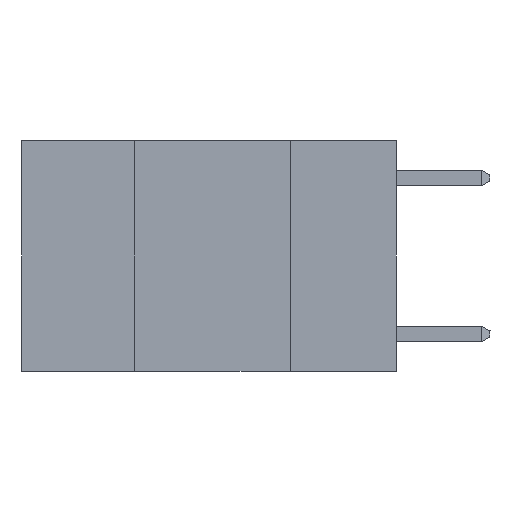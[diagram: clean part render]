
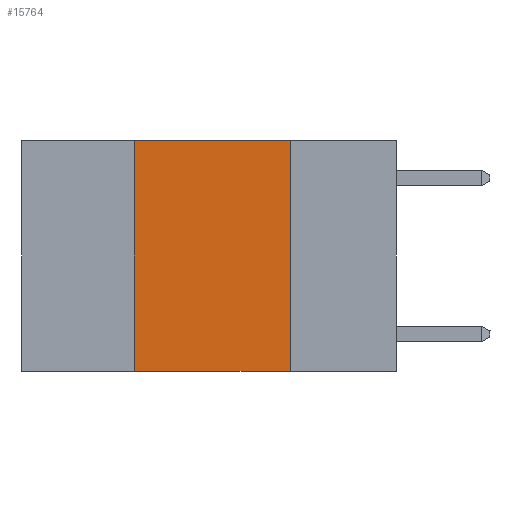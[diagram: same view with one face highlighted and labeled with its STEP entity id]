
A CAD part, left-side view. The second image highlights one B-rep face of the part: STEP entity #15764.
In plain terms, the highlighted planar face has unit normal (-1, 0, 0).
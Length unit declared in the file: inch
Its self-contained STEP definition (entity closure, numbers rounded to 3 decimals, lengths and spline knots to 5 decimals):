
#471 = CARTESIAN_POINT ( 'NONE',  ( 0., 0.6, 0. ) ) ;
#725 = VECTOR ( 'NONE', #10613, 39.37008 ) ;
#730 = VERTEX_POINT ( 'NONE', #13146 ) ;
#886 = CARTESIAN_POINT ( 'NONE',  ( 0., 0.6, -0.37 ) ) ;
#1570 = CARTESIAN_POINT ( 'NONE',  ( 0., 0.17, -0.37 ) ) ;
#1637 = ORIENTED_EDGE ( 'NONE', *, *, #3206, .T. ) ;
#1880 = CARTESIAN_POINT ( 'NONE',  ( 0., 0.17, 0. ) ) ;
#2827 = VERTEX_POINT ( 'NONE', #10248 ) ;
#3206 = EDGE_CURVE ( 'NONE', #8935, #9605, #15779, .T. ) ;
#3529 = DIRECTION ( 'NONE',  ( 0., 0., -1. ) ) ;
#4680 = FACE_OUTER_BOUND ( 'NONE', #5407, .T. ) ;
#5188 = CARTESIAN_POINT ( 'NONE',  ( 0., 0.42, 0. ) ) ;
#5199 = ORIENTED_EDGE ( 'NONE', *, *, #7371, .F. ) ;
#5407 = EDGE_LOOP ( 'NONE', ( #5199, #9253, #9108, #1637 ) ) ;
#5708 = DIRECTION ( 'NONE',  ( 0., 0., -1. ) ) ;
#6234 = DIRECTION ( 'NONE',  ( 0., -1., 0. ) ) ;
#6516 = LINE ( 'NONE', #5188, #725 ) ;
#7340 = DIRECTION ( 'NONE',  ( 1., 0., 0. ) ) ;
#7371 = EDGE_CURVE ( 'NONE', #730, #9605, #13830, .T. ) ;
#7540 = DIRECTION ( 'NONE',  ( 0., -1., 0. ) ) ;
#7768 = CARTESIAN_POINT ( 'NONE',  ( 0., 0.42, -0.37 ) ) ;
#8935 = VERTEX_POINT ( 'NONE', #7768 ) ;
#9108 = ORIENTED_EDGE ( 'NONE', *, *, #10853, .F. ) ;
#9253 = ORIENTED_EDGE ( 'NONE', *, *, #16695, .F. ) ;
#9605 = VERTEX_POINT ( 'NONE', #1570 ) ;
#10024 = PLANE ( 'NONE',  #12205 ) ;
#10248 = CARTESIAN_POINT ( 'NONE',  ( 0., 0.42, 0. ) ) ;
#10321 = CARTESIAN_POINT ( 'NONE',  ( 0., 0.6, 0. ) ) ;
#10613 = DIRECTION ( 'NONE',  ( 0., 0., 1. ) ) ;
#10853 = EDGE_CURVE ( 'NONE', #8935, #2827, #6516, .T. ) ;
#11704 = VECTOR ( 'NONE', #5708, 39.37008 ) ;
#12205 = AXIS2_PLACEMENT_3D ( 'NONE', #471, #7340, #3529 ) ;
#13146 = CARTESIAN_POINT ( 'NONE',  ( 0., 0.17, 0. ) ) ;
#13830 = LINE ( 'NONE', #1880, #11704 ) ;
#13912 = LINE ( 'NONE', #10321, #14514 ) ;
#14514 = VECTOR ( 'NONE', #6234, 39.37008 ) ;
#15764 = ADVANCED_FACE ( 'NONE', ( #4680 ), #10024, .F. ) ;
#15779 = LINE ( 'NONE', #886, #17473 ) ;
#16695 = EDGE_CURVE ( 'NONE', #2827, #730, #13912, .T. ) ;
#17473 = VECTOR ( 'NONE', #7540, 39.37008 ) ;
